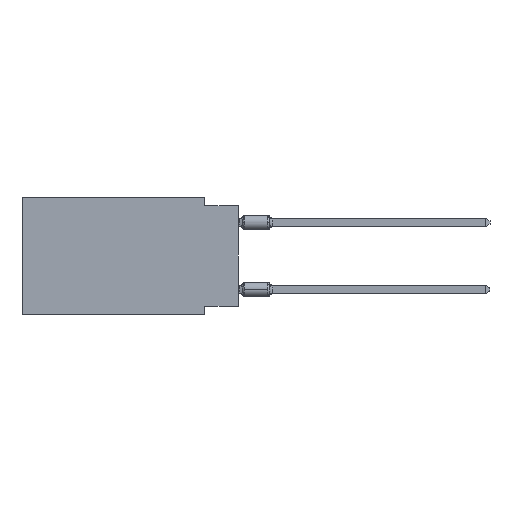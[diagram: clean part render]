
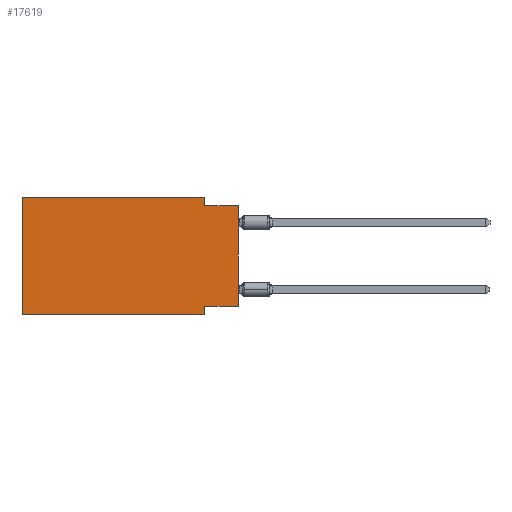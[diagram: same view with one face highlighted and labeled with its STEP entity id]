
A CAD part, left-side view. The second image highlights one B-rep face of the part: STEP entity #17619.
In plain terms, the highlighted planar face has unit normal (-1, 0, 0).
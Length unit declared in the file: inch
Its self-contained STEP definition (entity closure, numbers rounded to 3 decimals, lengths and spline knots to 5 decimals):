
#1157 = VERTEX_POINT ( 'NONE', #9238 ) ;
#1417 = VECTOR ( 'NONE', #13658, 39.37008 ) ;
#2257 = VERTEX_POINT ( 'NONE', #10912 ) ;
#2530 = VERTEX_POINT ( 'NONE', #14270 ) ;
#2734 = ORIENTED_EDGE ( 'NONE', *, *, #4053, .F. ) ;
#3431 = DIRECTION ( 'NONE',  ( 0., 0., -1. ) ) ;
#3444 = DIRECTION ( 'NONE',  ( 0., 0., 1. ) ) ;
#3456 = LINE ( 'NONE', #19785, #1417 ) ;
#3926 = DIRECTION ( 'NONE',  ( 0., 0., -1. ) ) ;
#4053 = EDGE_CURVE ( 'NONE', #22381, #9242, #13509, .T. ) ;
#5418 = CARTESIAN_POINT ( 'NONE',  ( 0., 0.1, -0.35 ) ) ;
#5661 = LINE ( 'NONE', #26248, #9287 ) ;
#7454 = CARTESIAN_POINT ( 'NONE',  ( 0., 0.645, 0. ) ) ;
#7959 = VECTOR ( 'NONE', #3444, 39.37008 ) ;
#8090 = FACE_OUTER_BOUND ( 'NONE', #12490, .T. ) ;
#8222 = DIRECTION ( 'NONE',  ( 0., 0., -1. ) ) ;
#8303 = CARTESIAN_POINT ( 'NONE',  ( 0., 0., 0. ) ) ;
#8880 = DIRECTION ( 'NONE',  ( 0., -1., 0. ) ) ;
#9008 = CARTESIAN_POINT ( 'NONE',  ( 0., 0.645, -0.35 ) ) ;
#9129 = VECTOR ( 'NONE', #17396, 39.37008 ) ;
#9238 = CARTESIAN_POINT ( 'NONE',  ( 0., 0.645, 0. ) ) ;
#9242 = VERTEX_POINT ( 'NONE', #19976 ) ;
#9287 = VECTOR ( 'NONE', #3926, 39.37008 ) ;
#9314 = CARTESIAN_POINT ( 'NONE',  ( 0., 0.645, 0. ) ) ;
#9850 = ORIENTED_EDGE ( 'NONE', *, *, #21670, .F. ) ;
#10181 = VECTOR ( 'NONE', #13518, 39.37008 ) ;
#10689 = CARTESIAN_POINT ( 'NONE',  ( 0., 0.645, -0.35 ) ) ;
#10912 = CARTESIAN_POINT ( 'NONE',  ( 0., 0., -0.325 ) ) ;
#11439 = EDGE_CURVE ( 'NONE', #15710, #18642, #5661, .T. ) ;
#11802 = LINE ( 'NONE', #7454, #7959 ) ;
#12157 = AXIS2_PLACEMENT_3D ( 'NONE', #12170, #20037, #8222 ) ;
#12170 = CARTESIAN_POINT ( 'NONE',  ( 0., 0.645, 0. ) ) ;
#12490 = EDGE_LOOP ( 'NONE', ( #16573, #9850, #2734, #19699, #24449, #13119, #20805, #18972 ) ) ;
#13119 = ORIENTED_EDGE ( 'NONE', *, *, #14864, .T. ) ;
#13190 = EDGE_CURVE ( 'NONE', #2257, #15710, #25641, .T. ) ;
#13509 = LINE ( 'NONE', #21623, #23798 ) ;
#13518 = DIRECTION ( 'NONE',  ( 0., 1., 0. ) ) ;
#13658 = DIRECTION ( 'NONE',  ( 0., -1., 0. ) ) ;
#14270 = CARTESIAN_POINT ( 'NONE',  ( 0., 0., -0.025 ) ) ;
#14864 = EDGE_CURVE ( 'NONE', #25567, #18642, #16841, .T. ) ;
#15524 = CARTESIAN_POINT ( 'NONE',  ( 0., 0., -0.325 ) ) ;
#15710 = VERTEX_POINT ( 'NONE', #15804 ) ;
#15804 = CARTESIAN_POINT ( 'NONE',  ( 0., 0.1, -0.325 ) ) ;
#16573 = ORIENTED_EDGE ( 'NONE', *, *, #19370, .T. ) ;
#16841 = LINE ( 'NONE', #9008, #20929 ) ;
#17396 = DIRECTION ( 'NONE',  ( 0., -1., 0. ) ) ;
#17479 = EDGE_CURVE ( 'NONE', #25567, #1157, #11802, .T. ) ;
#17619 = ADVANCED_FACE ( 'NONE', ( #8090 ), #24548, .F. ) ;
#18595 = VECTOR ( 'NONE', #21033, 39.37008 ) ;
#18642 = VERTEX_POINT ( 'NONE', #5418 ) ;
#18972 = ORIENTED_EDGE ( 'NONE', *, *, #13190, .F. ) ;
#19370 = EDGE_CURVE ( 'NONE', #2257, #2530, #20636, .T. ) ;
#19699 = ORIENTED_EDGE ( 'NONE', *, *, #24724, .F. ) ;
#19785 = CARTESIAN_POINT ( 'NONE',  ( 0., 0., -0.025 ) ) ;
#19976 = CARTESIAN_POINT ( 'NONE',  ( 0., 0.1, -0.025 ) ) ;
#20037 = DIRECTION ( 'NONE',  ( 1., 0., 0. ) ) ;
#20622 = CARTESIAN_POINT ( 'NONE',  ( 0., 0.1, 0. ) ) ;
#20636 = LINE ( 'NONE', #8303, #18595 ) ;
#20805 = ORIENTED_EDGE ( 'NONE', *, *, #11439, .F. ) ;
#20929 = VECTOR ( 'NONE', #8880, 39.37008 ) ;
#21033 = DIRECTION ( 'NONE',  ( 0., 0., 1. ) ) ;
#21117 = LINE ( 'NONE', #9314, #9129 ) ;
#21623 = CARTESIAN_POINT ( 'NONE',  ( 0., 0.1, 0. ) ) ;
#21670 = EDGE_CURVE ( 'NONE', #9242, #2530, #3456, .T. ) ;
#22381 = VERTEX_POINT ( 'NONE', #20622 ) ;
#23798 = VECTOR ( 'NONE', #3431, 39.37008 ) ;
#24449 = ORIENTED_EDGE ( 'NONE', *, *, #17479, .F. ) ;
#24548 = PLANE ( 'NONE',  #12157 ) ;
#24724 = EDGE_CURVE ( 'NONE', #1157, #22381, #21117, .T. ) ;
#25567 = VERTEX_POINT ( 'NONE', #10689 ) ;
#25641 = LINE ( 'NONE', #15524, #10181 ) ;
#26248 = CARTESIAN_POINT ( 'NONE',  ( 0., 0.1, -0.35 ) ) ;
